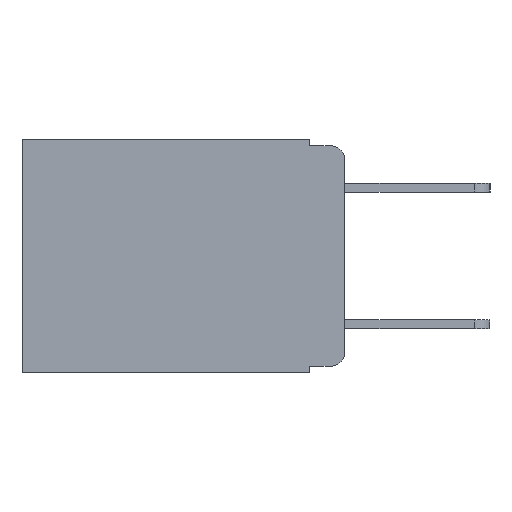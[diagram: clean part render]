
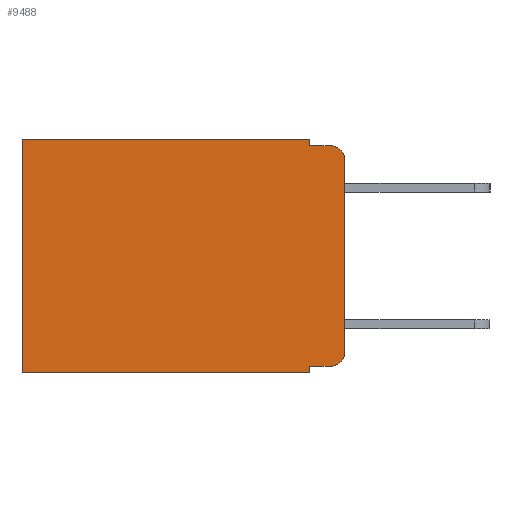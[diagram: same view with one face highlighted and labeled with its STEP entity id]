
A CAD part, left-side view. The second image highlights one B-rep face of the part: STEP entity #9488.
In plain terms, the highlighted planar face has unit normal (-1, 0, 0).
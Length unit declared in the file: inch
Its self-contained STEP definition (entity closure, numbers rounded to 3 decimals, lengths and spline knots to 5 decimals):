
#97 = AXIS2_PLACEMENT_3D ( 'NONE', #6747, #12369, #18539 ) ;
#273 = CARTESIAN_POINT ( 'NONE',  ( 0.298, 0., -0.03 ) ) ;
#418 = CARTESIAN_POINT ( 'NONE',  ( 0.298, 0.051, -0.333 ) ) ;
#504 = EDGE_CURVE ( 'NONE', #12705, #6958, #17392, .T. ) ;
#612 = EDGE_CURVE ( 'NONE', #8430, #3487, #17953, .T. ) ;
#657 = CARTESIAN_POINT ( 'NONE',  ( 0.298, 0.473, -0.343 ) ) ;
#763 = ORIENTED_EDGE ( 'NONE', *, *, #16919, .F. ) ;
#819 = ORIENTED_EDGE ( 'NONE', *, *, #612, .T. ) ;
#875 = VERTEX_POINT ( 'NONE', #7022 ) ;
#945 = ORIENTED_EDGE ( 'NONE', *, *, #989, .F. ) ;
#989 = EDGE_CURVE ( 'NONE', #8626, #3487, #6757, .T. ) ;
#1007 = EDGE_CURVE ( 'NONE', #10441, #8146, #10310, .T. ) ;
#1349 = ORIENTED_EDGE ( 'NONE', *, *, #9111, .F. ) ;
#1393 = ORIENTED_EDGE ( 'NONE', *, *, #1007, .T. ) ;
#1394 = FACE_OUTER_BOUND ( 'NONE', #1733, .T. ) ;
#1413 = ORIENTED_EDGE ( 'NONE', *, *, #7332, .T. ) ;
#1498 = ORIENTED_EDGE ( 'NONE', *, *, #2790, .F. ) ;
#1558 = ORIENTED_EDGE ( 'NONE', *, *, #5920, .F. ) ;
#1602 = ORIENTED_EDGE ( 'NONE', *, *, #12088, .T. ) ;
#1733 = EDGE_LOOP ( 'NONE', ( #763, #819, #945, #1349, #1393, #1413, #1498, #1558, #1602, #1742 ) ) ;
#1742 = ORIENTED_EDGE ( 'NONE', *, *, #504, .T. ) ;
#2312 = DIRECTION ( 'NONE',  ( 0., 0., -1. ) ) ;
#2790 = EDGE_CURVE ( 'NONE', #875, #11404, #7166, .T. ) ;
#2844 = LINE ( 'NONE', #9974, #7073 ) ;
#3309 = DIRECTION ( 'NONE',  ( -1., 0., 0. ) ) ;
#3314 = VECTOR ( 'NONE', #7223, 39.37008 ) ;
#3487 = VERTEX_POINT ( 'NONE', #12364 ) ;
#3655 = DIRECTION ( 'NONE',  ( 0., 0., -1. ) ) ;
#3769 = CARTESIAN_POINT ( 'NONE',  ( 0.298, 0.473, 0. ) ) ;
#4196 = LINE ( 'NONE', #9019, #18887 ) ;
#4894 = DIRECTION ( 'NONE',  ( 0., -1., 0. ) ) ;
#5473 = DIRECTION ( 'NONE',  ( 0., 1., 0. ) ) ;
#5614 = CARTESIAN_POINT ( 'NONE',  ( 0.298, 0.02, -0.333 ) ) ;
#5920 = EDGE_CURVE ( 'NONE', #12044, #875, #18610, .T. ) ;
#6283 = VECTOR ( 'NONE', #5473, 39.37008 ) ;
#6565 = CARTESIAN_POINT ( 'NONE',  ( 0.298, 0.02, -0.313 ) ) ;
#6601 = AXIS2_PLACEMENT_3D ( 'NONE', #9863, #12636, #3655 ) ;
#6747 = CARTESIAN_POINT ( 'NONE',  ( 0.298, 0.02, -0.03 ) ) ;
#6757 = LINE ( 'NONE', #13019, #17936 ) ;
#6796 = PLANE ( 'NONE',  #6601 ) ;
#6929 = DIRECTION ( 'NONE',  ( 0., -1., 0. ) ) ;
#6958 = VERTEX_POINT ( 'NONE', #13473 ) ;
#7022 = CARTESIAN_POINT ( 'NONE',  ( 0.298, 0.051, -0.343 ) ) ;
#7046 = AXIS2_PLACEMENT_3D ( 'NONE', #6565, #3309, #9429 ) ;
#7073 = VECTOR ( 'NONE', #6929, 39.37008 ) ;
#7166 = LINE ( 'NONE', #13844, #10672 ) ;
#7202 = CARTESIAN_POINT ( 'NONE',  ( 0.298, 0.051, -0.01 ) ) ;
#7223 = DIRECTION ( 'NONE',  ( 0., 0., -1. ) ) ;
#7332 = EDGE_CURVE ( 'NONE', #8146, #11404, #7993, .T. ) ;
#7504 = DIRECTION ( 'NONE',  ( 0., 0., -1. ) ) ;
#7993 = LINE ( 'NONE', #3769, #18146 ) ;
#8141 = CARTESIAN_POINT ( 'NONE',  ( 0.298, 0., 0. ) ) ;
#8146 = VERTEX_POINT ( 'NONE', #13502 ) ;
#8296 = CARTESIAN_POINT ( 'NONE',  ( 0.298, 0., 0. ) ) ;
#8414 = LINE ( 'NONE', #8141, #15470 ) ;
#8430 = VERTEX_POINT ( 'NONE', #273 ) ;
#8626 = VERTEX_POINT ( 'NONE', #7202 ) ;
#9019 = CARTESIAN_POINT ( 'NONE',  ( 0.298, 0.051, 0. ) ) ;
#9111 = EDGE_CURVE ( 'NONE', #10441, #8626, #4196, .T. ) ;
#9210 = DIRECTION ( 'NONE',  ( 0., 1., 0. ) ) ;
#9429 = DIRECTION ( 'NONE',  ( 0., 0., -1. ) ) ;
#9488 = ADVANCED_FACE ( 'NONE', ( #1394 ), #6796, .F. ) ;
#9656 = DIRECTION ( 'NONE',  ( 0., 0., -1. ) ) ;
#9863 = CARTESIAN_POINT ( 'NONE',  ( 0.298, 0., 0. ) ) ;
#9974 = CARTESIAN_POINT ( 'NONE',  ( 0.298, 0.051, -0.333 ) ) ;
#10310 = LINE ( 'NONE', #8296, #6283 ) ;
#10441 = VERTEX_POINT ( 'NONE', #16299 ) ;
#10672 = VECTOR ( 'NONE', #9210, 39.37008 ) ;
#11404 = VERTEX_POINT ( 'NONE', #657 ) ;
#12044 = VERTEX_POINT ( 'NONE', #418 ) ;
#12088 = EDGE_CURVE ( 'NONE', #12044, #12705, #2844, .T. ) ;
#12364 = CARTESIAN_POINT ( 'NONE',  ( 0.298, 0.02, -0.01 ) ) ;
#12369 = DIRECTION ( 'NONE',  ( -1., 0., 0. ) ) ;
#12636 = DIRECTION ( 'NONE',  ( 1., 0., 0. ) ) ;
#12705 = VERTEX_POINT ( 'NONE', #5614 ) ;
#13019 = CARTESIAN_POINT ( 'NONE',  ( 0.298, 0.051, -0.01 ) ) ;
#13473 = CARTESIAN_POINT ( 'NONE',  ( 0.298, 0., -0.313 ) ) ;
#13502 = CARTESIAN_POINT ( 'NONE',  ( 0.298, 0.473, 0. ) ) ;
#13844 = CARTESIAN_POINT ( 'NONE',  ( 0.298, 0., -0.343 ) ) ;
#15470 = VECTOR ( 'NONE', #9656, 39.37008 ) ;
#16299 = CARTESIAN_POINT ( 'NONE',  ( 0.298, 0.051, 0. ) ) ;
#16919 = EDGE_CURVE ( 'NONE', #8430, #6958, #8414, .T. ) ;
#17012 = CARTESIAN_POINT ( 'NONE',  ( 0.298, 0.051, 0. ) ) ;
#17392 = CIRCLE ( 'NONE', #7046, 0.02 ) ;
#17936 = VECTOR ( 'NONE', #4894, 39.37008 ) ;
#17953 = CIRCLE ( 'NONE', #97, 0.02 ) ;
#18146 = VECTOR ( 'NONE', #2312, 39.37008 ) ;
#18539 = DIRECTION ( 'NONE',  ( 0., 0., -1. ) ) ;
#18610 = LINE ( 'NONE', #17012, #3314 ) ;
#18887 = VECTOR ( 'NONE', #7504, 39.37008 ) ;
